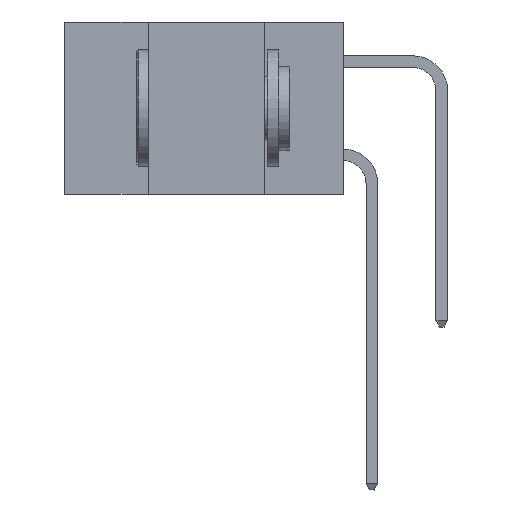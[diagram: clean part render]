
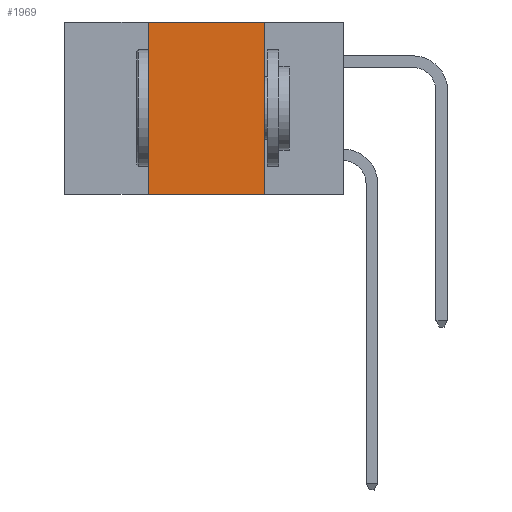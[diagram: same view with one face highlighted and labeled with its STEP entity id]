
A CAD part, left-side view. The second image highlights one B-rep face of the part: STEP entity #1969.
In plain terms, the highlighted planar face has unit normal (-1, 0, 0).
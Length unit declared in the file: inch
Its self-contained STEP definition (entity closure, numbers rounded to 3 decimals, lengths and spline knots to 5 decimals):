
#398 = CARTESIAN_POINT ( 'NONE',  ( 0., 0.17, -0.37 ) ) ;
#1183 = DIRECTION ( 'NONE',  ( 0., -1., 0. ) ) ;
#1885 = CARTESIAN_POINT ( 'NONE',  ( 0., 0.17, 0. ) ) ;
#1969 = ADVANCED_FACE ( 'NONE', ( #3426 ), #3454, .F. ) ;
#2175 = VECTOR ( 'NONE', #15193, 39.37008 ) ;
#3391 = DIRECTION ( 'NONE',  ( 0., 0., -1. ) ) ;
#3426 = FACE_OUTER_BOUND ( 'NONE', #12485, .T. ) ;
#3454 = PLANE ( 'NONE',  #10164 ) ;
#3513 = CARTESIAN_POINT ( 'NONE',  ( 0., 0.17, 0. ) ) ;
#3514 = ORIENTED_EDGE ( 'NONE', *, *, #8124, .F. ) ;
#4118 = CARTESIAN_POINT ( 'NONE',  ( 0., 0.42, 0. ) ) ;
#4242 = EDGE_CURVE ( 'NONE', #12049, #13658, #13202, .T. ) ;
#4406 = VECTOR ( 'NONE', #8087, 39.37008 ) ;
#5250 = VECTOR ( 'NONE', #1183, 39.37008 ) ;
#5519 = VERTEX_POINT ( 'NONE', #9010 ) ;
#5530 = CARTESIAN_POINT ( 'NONE',  ( 0., 0.42, -0.37 ) ) ;
#5544 = LINE ( 'NONE', #1885, #2175 ) ;
#6013 = CARTESIAN_POINT ( 'NONE',  ( 0., 0.6, 0. ) ) ;
#8087 = DIRECTION ( 'NONE',  ( 0., 0., 1. ) ) ;
#8124 = EDGE_CURVE ( 'NONE', #12049, #5519, #13350, .T. ) ;
#8711 = CARTESIAN_POINT ( 'NONE',  ( 0., 0.6, -0.37 ) ) ;
#8933 = VECTOR ( 'NONE', #11670, 39.37008 ) ;
#9010 = CARTESIAN_POINT ( 'NONE',  ( 0., 0.42, 0. ) ) ;
#9205 = VERTEX_POINT ( 'NONE', #3513 ) ;
#9638 = EDGE_CURVE ( 'NONE', #9205, #13658, #5544, .T. ) ;
#9923 = LINE ( 'NONE', #11844, #8933 ) ;
#10164 = AXIS2_PLACEMENT_3D ( 'NONE', #6013, #13673, #3391 ) ;
#10348 = ORIENTED_EDGE ( 'NONE', *, *, #4242, .T. ) ;
#11670 = DIRECTION ( 'NONE',  ( 0., -1., 0. ) ) ;
#11844 = CARTESIAN_POINT ( 'NONE',  ( 0., 0.6, 0. ) ) ;
#12049 = VERTEX_POINT ( 'NONE', #5530 ) ;
#12485 = EDGE_LOOP ( 'NONE', ( #14867, #16060, #3514, #10348 ) ) ;
#13202 = LINE ( 'NONE', #8711, #5250 ) ;
#13350 = LINE ( 'NONE', #4118, #4406 ) ;
#13658 = VERTEX_POINT ( 'NONE', #398 ) ;
#13673 = DIRECTION ( 'NONE',  ( 1., 0., 0. ) ) ;
#14258 = EDGE_CURVE ( 'NONE', #5519, #9205, #9923, .T. ) ;
#14867 = ORIENTED_EDGE ( 'NONE', *, *, #9638, .F. ) ;
#15193 = DIRECTION ( 'NONE',  ( 0., 0., -1. ) ) ;
#16060 = ORIENTED_EDGE ( 'NONE', *, *, #14258, .F. ) ;
